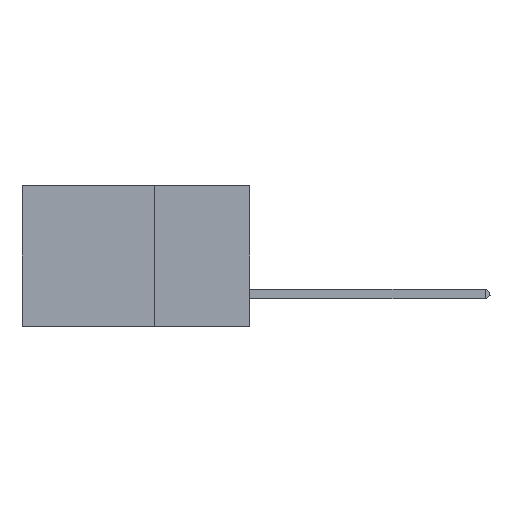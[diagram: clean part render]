
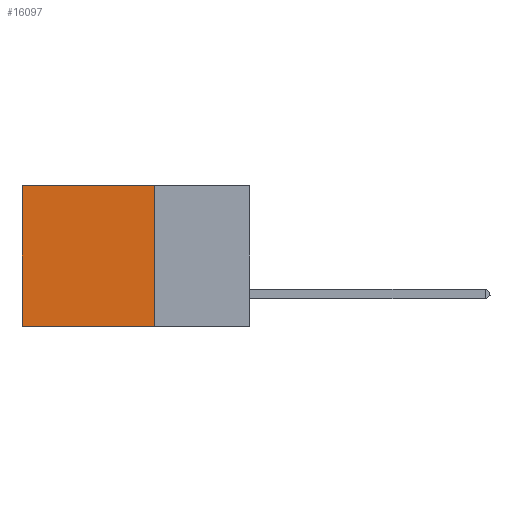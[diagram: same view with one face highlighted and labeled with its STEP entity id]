
A CAD part, left-side view. The second image highlights one B-rep face of the part: STEP entity #16097.
In plain terms, the highlighted planar face has unit normal (-1, 0, 0).
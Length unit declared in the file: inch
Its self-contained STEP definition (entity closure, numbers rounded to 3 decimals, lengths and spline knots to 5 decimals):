
#318 = EDGE_CURVE ( 'NONE', #12075, #10533, #5963, .T. ) ;
#1651 = VECTOR ( 'NONE', #15668, 39.37008 ) ;
#1926 = EDGE_CURVE ( 'NONE', #10707, #10533, #2056, .T. ) ;
#2017 = PLANE ( 'NONE',  #13001 ) ;
#2056 = LINE ( 'NONE', #6631, #1651 ) ;
#2156 = LINE ( 'NONE', #2613, #14885 ) ;
#2516 = VECTOR ( 'NONE', #10343, 39.37008 ) ;
#2613 = CARTESIAN_POINT ( 'NONE',  ( 0.2875, 0.25, 0. ) ) ;
#2831 = CARTESIAN_POINT ( 'NONE',  ( 0.2875, 0.25, -0.37 ) ) ;
#3085 = VERTEX_POINT ( 'NONE', #6009 ) ;
#4995 = CARTESIAN_POINT ( 'NONE',  ( 0.2875, 0.25, 0. ) ) ;
#5035 = EDGE_CURVE ( 'NONE', #3085, #10707, #15243, .T. ) ;
#5289 = CARTESIAN_POINT ( 'NONE',  ( 0.2875, 0.6, -0.37 ) ) ;
#5428 = ORIENTED_EDGE ( 'NONE', *, *, #318, .F. ) ;
#5963 = LINE ( 'NONE', #2831, #2516 ) ;
#6009 = CARTESIAN_POINT ( 'NONE',  ( 0.2875, 0.25, 0. ) ) ;
#6631 = CARTESIAN_POINT ( 'NONE',  ( 0.2875, 0.6, 0. ) ) ;
#7199 = DIRECTION ( 'NONE',  ( 0., 0., -1. ) ) ;
#8133 = FACE_OUTER_BOUND ( 'NONE', #15801, .T. ) ;
#9243 = EDGE_CURVE ( 'NONE', #3085, #12075, #2156, .T. ) ;
#10153 = ORIENTED_EDGE ( 'NONE', *, *, #5035, .T. ) ;
#10249 = DIRECTION ( 'NONE',  ( 0., 0., -1. ) ) ;
#10343 = DIRECTION ( 'NONE',  ( 0., 1., 0. ) ) ;
#10533 = VERTEX_POINT ( 'NONE', #5289 ) ;
#10707 = VERTEX_POINT ( 'NONE', #12038 ) ;
#11924 = CARTESIAN_POINT ( 'NONE',  ( 0.2875, 0.25, -0.37 ) ) ;
#12038 = CARTESIAN_POINT ( 'NONE',  ( 0.2875, 0.6, 0. ) ) ;
#12075 = VERTEX_POINT ( 'NONE', #11924 ) ;
#13001 = AXIS2_PLACEMENT_3D ( 'NONE', #13621, #13565, #7199 ) ;
#13565 = DIRECTION ( 'NONE',  ( 1., 0., 0. ) ) ;
#13607 = ORIENTED_EDGE ( 'NONE', *, *, #1926, .T. ) ;
#13621 = CARTESIAN_POINT ( 'NONE',  ( 0.2875, 0.25, 0. ) ) ;
#14089 = ORIENTED_EDGE ( 'NONE', *, *, #9243, .F. ) ;
#14885 = VECTOR ( 'NONE', #10249, 39.37008 ) ;
#15243 = LINE ( 'NONE', #4995, #15451 ) ;
#15266 = DIRECTION ( 'NONE',  ( 0., 1., 0. ) ) ;
#15451 = VECTOR ( 'NONE', #15266, 39.37008 ) ;
#15668 = DIRECTION ( 'NONE',  ( 0., 0., -1. ) ) ;
#15801 = EDGE_LOOP ( 'NONE', ( #13607, #5428, #14089, #10153 ) ) ;
#16097 = ADVANCED_FACE ( 'NONE', ( #8133 ), #2017, .F. ) ;
